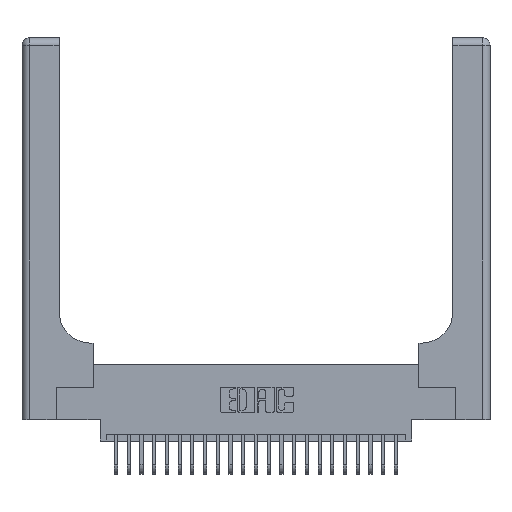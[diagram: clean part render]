
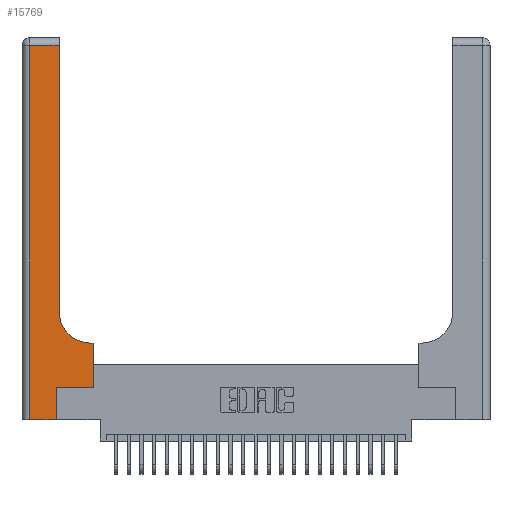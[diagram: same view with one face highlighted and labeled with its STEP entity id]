
A CAD part, top view. The second image highlights one B-rep face of the part: STEP entity #15769.
In plain terms, the highlighted planar face has unit normal (0, 0, 1).
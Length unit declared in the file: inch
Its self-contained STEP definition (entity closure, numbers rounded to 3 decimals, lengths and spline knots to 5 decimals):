
#424 = ORIENTED_EDGE ( 'NONE', *, *, #14327, .T. ) ;
#677 = LINE ( 'NONE', #8878, #11474 ) ;
#1295 = EDGE_CURVE ( 'NONE', #14858, #12645, #7576, .T. ) ;
#1724 = EDGE_CURVE ( 'NONE', #7740, #14858, #9545, .T. ) ;
#1785 = VECTOR ( 'NONE', #20816, 39.37008 ) ;
#3107 = CIRCLE ( 'NONE', #19491, 0.25 ) ;
#3640 = DIRECTION ( 'NONE',  ( 1., 0., 0. ) ) ;
#3820 = VECTOR ( 'NONE', #14184, 39.37008 ) ;
#4630 = PLANE ( 'NONE',  #23777 ) ;
#4809 = EDGE_LOOP ( 'NONE', ( #12370, #17119, #17908, #14835, #8325, #9436, #424, #5422, #20439 ) ) ;
#5049 = VECTOR ( 'NONE', #12154, 39.37008 ) ;
#5422 = ORIENTED_EDGE ( 'NONE', *, *, #13859, .T. ) ;
#5598 = VECTOR ( 'NONE', #18397, 39.37008 ) ;
#5633 = CARTESIAN_POINT ( 'NONE',  ( 0.269, 0.25, 0.37 ) ) ;
#5873 = CARTESIAN_POINT ( 'NONE',  ( 0.5415, 0.85, 0.37 ) ) ;
#6364 = FACE_OUTER_BOUND ( 'NONE', #4809, .T. ) ;
#6822 = CARTESIAN_POINT ( 'NONE',  ( 0., 3., 0.37 ) ) ;
#7576 = LINE ( 'NONE', #23270, #18202 ) ;
#7740 = VERTEX_POINT ( 'NONE', #14822 ) ;
#7820 = CARTESIAN_POINT ( 'NONE',  ( 0., 2.94, 0.37 ) ) ;
#8031 = DIRECTION ( 'NONE',  ( 1., 0., 0. ) ) ;
#8256 = EDGE_CURVE ( 'NONE', #9017, #26311, #22505, .T. ) ;
#8310 = DIRECTION ( 'NONE',  ( 0., 1., 0. ) ) ;
#8325 = ORIENTED_EDGE ( 'NONE', *, *, #1724, .T. ) ;
#8338 = CARTESIAN_POINT ( 'NONE',  ( 0.5585, 0.6, 0.37 ) ) ;
#8878 = CARTESIAN_POINT ( 'NONE',  ( 0.2915, 0.6, 0.37 ) ) ;
#8957 = DIRECTION ( 'NONE',  ( 0., 0., -1. ) ) ;
#9017 = VERTEX_POINT ( 'NONE', #25583 ) ;
#9149 = CARTESIAN_POINT ( 'NONE',  ( 0.06, 2.94, 0.37 ) ) ;
#9436 = ORIENTED_EDGE ( 'NONE', *, *, #1295, .T. ) ;
#9545 = LINE ( 'NONE', #14523, #3820 ) ;
#10467 = EDGE_CURVE ( 'NONE', #22021, #23162, #3107, .T. ) ;
#10942 = DIRECTION ( 'NONE',  ( -1., 0., 0. ) ) ;
#11474 = VECTOR ( 'NONE', #10942, 39.37008 ) ;
#11696 = EDGE_CURVE ( 'NONE', #23162, #9017, #17736, .T. ) ;
#12154 = DIRECTION ( 'NONE',  ( 0., 1., 0. ) ) ;
#12305 = CARTESIAN_POINT ( 'NONE',  ( 0.2915, 0.85, 0.37 ) ) ;
#12370 = ORIENTED_EDGE ( 'NONE', *, *, #11696, .T. ) ;
#12645 = VERTEX_POINT ( 'NONE', #23509 ) ;
#13199 = LINE ( 'NONE', #18711, #1785 ) ;
#13450 = LINE ( 'NONE', #20968, #23297 ) ;
#13859 = EDGE_CURVE ( 'NONE', #24453, #22021, #677, .T. ) ;
#14184 = DIRECTION ( 'NONE',  ( 0., 1., 0. ) ) ;
#14327 = EDGE_CURVE ( 'NONE', #12645, #24453, #13450, .T. ) ;
#14523 = CARTESIAN_POINT ( 'NONE',  ( 0.269, 0., 0.37 ) ) ;
#14822 = CARTESIAN_POINT ( 'NONE',  ( 0.269, 0., 0.37 ) ) ;
#14835 = ORIENTED_EDGE ( 'NONE', *, *, #23661, .T. ) ;
#14858 = VERTEX_POINT ( 'NONE', #5633 ) ;
#15769 = ADVANCED_FACE ( 'NONE', ( #6364 ), #4630, .F. ) ;
#16006 = VECTOR ( 'NONE', #3640, 39.37008 ) ;
#16696 = LINE ( 'NONE', #22671, #16006 ) ;
#17119 = ORIENTED_EDGE ( 'NONE', *, *, #8256, .T. ) ;
#17736 = LINE ( 'NONE', #24783, #5049 ) ;
#17908 = ORIENTED_EDGE ( 'NONE', *, *, #20339, .T. ) ;
#18202 = VECTOR ( 'NONE', #23552, 39.37008 ) ;
#18397 = DIRECTION ( 'NONE',  ( -1., 0., 0. ) ) ;
#18711 = CARTESIAN_POINT ( 'NONE',  ( 0.06, 3., 0.37 ) ) ;
#19491 = AXIS2_PLACEMENT_3D ( 'NONE', #5873, #20704, #8031 ) ;
#20339 = EDGE_CURVE ( 'NONE', #26311, #24272, #13199, .T. ) ;
#20439 = ORIENTED_EDGE ( 'NONE', *, *, #10467, .T. ) ;
#20704 = DIRECTION ( 'NONE',  ( 0., 0., -1. ) ) ;
#20816 = DIRECTION ( 'NONE',  ( 0., -1., 0. ) ) ;
#20968 = CARTESIAN_POINT ( 'NONE',  ( 0.5585, 0.25, 0.37 ) ) ;
#22021 = VERTEX_POINT ( 'NONE', #22189 ) ;
#22189 = CARTESIAN_POINT ( 'NONE',  ( 0.5415, 0.6, 0.37 ) ) ;
#22505 = LINE ( 'NONE', #7820, #5598 ) ;
#22671 = CARTESIAN_POINT ( 'NONE',  ( 0., 0., 0.37 ) ) ;
#23162 = VERTEX_POINT ( 'NONE', #12305 ) ;
#23270 = CARTESIAN_POINT ( 'NONE',  ( 0.269, 0.25, 0.37 ) ) ;
#23297 = VECTOR ( 'NONE', #8310, 39.37008 ) ;
#23509 = CARTESIAN_POINT ( 'NONE',  ( 0.5585, 0.25, 0.37 ) ) ;
#23552 = DIRECTION ( 'NONE',  ( 1., 0., 0. ) ) ;
#23661 = EDGE_CURVE ( 'NONE', #24272, #7740, #16696, .T. ) ;
#23722 = DIRECTION ( 'NONE',  ( -1., 0., 0. ) ) ;
#23777 = AXIS2_PLACEMENT_3D ( 'NONE', #6822, #8957, #23722 ) ;
#24272 = VERTEX_POINT ( 'NONE', #26734 ) ;
#24453 = VERTEX_POINT ( 'NONE', #8338 ) ;
#24783 = CARTESIAN_POINT ( 'NONE',  ( 0.2915, 3., 0.37 ) ) ;
#25583 = CARTESIAN_POINT ( 'NONE',  ( 0.2915, 2.94, 0.37 ) ) ;
#26311 = VERTEX_POINT ( 'NONE', #9149 ) ;
#26734 = CARTESIAN_POINT ( 'NONE',  ( 0.06, 0., 0.37 ) ) ;
